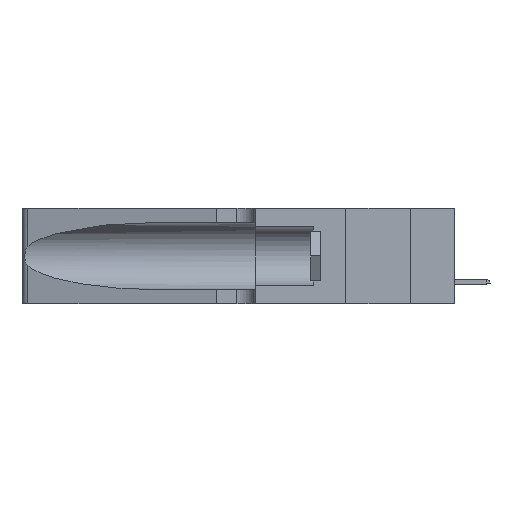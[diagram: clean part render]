
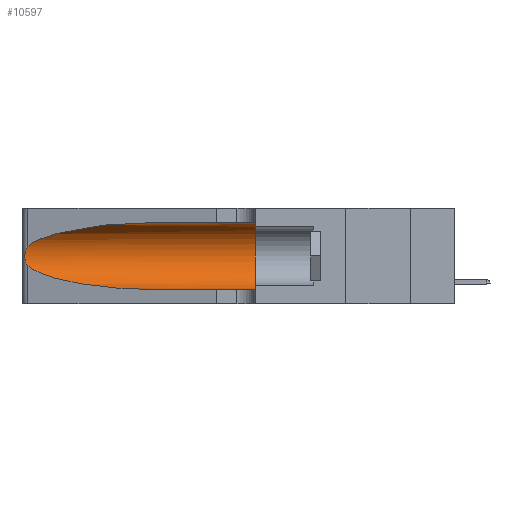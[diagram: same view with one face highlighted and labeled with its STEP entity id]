
A CAD part, left-side view. The second image highlights one B-rep face of the part: STEP entity #10597.
In plain terms, the highlighted cylindrical face has radius 3.308 mm (diameter 6.617 mm), a partial arc.
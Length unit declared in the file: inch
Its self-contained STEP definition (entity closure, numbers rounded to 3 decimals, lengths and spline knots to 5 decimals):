
#1844 = ORIENTED_EDGE ( 'NONE', *, *, #12029, .T. ) ;
#2015 = CARTESIAN_POINT ( 'NONE',  ( 0.25487, 1.22718, 0.22369 ) ) ;
#2252 = CARTESIAN_POINT ( 'NONE',  ( 0.26017, 1.23833, 0.17102 ) ) ;
#2272 = DIRECTION ( 'NONE',  ( 0., -1., 0. ) ) ;
#3058 =( BOUNDED_CURVE ( )  B_SPLINE_CURVE ( 3, ( #35166, #35877, #16623, #16371 ),
 .UNSPECIFIED., .F., .F. ) 
 B_SPLINE_CURVE_WITH_KNOTS ( ( 4, 4 ),
 ( 3.44316, 4.71239 ),
 .UNSPECIFIED. ) 
 CURVE ( )  GEOMETRIC_REPRESENTATION_ITEM ( )  RATIONAL_B_SPLINE_CURVE ( ( 1., 0.87, 0.87, 1. ) ) 
 REPRESENTATION_ITEM ( '' )  );
#3721 = DIRECTION ( 'NONE',  ( 0., 0., -1. ) ) ;
#3749 = EDGE_CURVE ( 'NONE', #28624, #7255, #40687, .T. ) ;
#4473 = CARTESIAN_POINT ( 'NONE',  ( 0.25487, 1.22718, 0.22369 ) ) ;
#4740 = CARTESIAN_POINT ( 'NONE',  ( 0.25487, 1.22718, 0.14631 ) ) ;
#5565 = AXIS2_PLACEMENT_3D ( 'NONE', #10467, #25495, #40591 ) ;
#5703 = EDGE_CURVE ( 'NONE', #43913, #32216, #21522, .T. ) ;
#6181 = AXIS2_PLACEMENT_3D ( 'NONE', #15055, #29634, #3721 ) ;
#6651 = CARTESIAN_POINT ( 'NONE',  ( 0.1305, 0.35, 0.05475 ) ) ;
#6897 = EDGE_CURVE ( 'NONE', #7255, #42079, #3058, .T. ) ;
#7200 = CIRCLE ( 'NONE', #5565, 0.13025 ) ;
#7255 = VERTEX_POINT ( 'NONE', #4740 ) ;
#9698 = CARTESIAN_POINT ( 'NONE',  ( 0.25854, 1.2359, 0.20912 ) ) ;
#9940 = CARTESIAN_POINT ( 'NONE',  ( 0.25555, 1.22993, 0.14849 ) ) ;
#10467 = CARTESIAN_POINT ( 'NONE',  ( 0.1305, 0.35, 0.185 ) ) ;
#10597 = ADVANCED_FACE ( 'NONE', ( #14576 ), #15294, .F. ) ;
#10708 = CARTESIAN_POINT ( 'NONE',  ( 0.1305, 1.61858, 0.31525 ) ) ;
#11825 = CARTESIAN_POINT ( 'NONE',  ( 0.2373, 1.15595, 0.28018 ) ) ;
#12029 = EDGE_CURVE ( 'NONE', #42079, #45597, #19730, .T. ) ;
#12962 = VECTOR ( 'NONE', #2272, 39.37008 ) ;
#14576 = FACE_OUTER_BOUND ( 'NONE', #19573, .T. ) ;
#15055 = CARTESIAN_POINT ( 'NONE',  ( 0.1305, 1.61858, 0.185 ) ) ;
#15294 = CYLINDRICAL_SURFACE ( 'NONE', #6181, 0.13025 ) ;
#16371 = CARTESIAN_POINT ( 'NONE',  ( 0.1305, 0.72297, 0.05475 ) ) ;
#16623 = CARTESIAN_POINT ( 'NONE',  ( 0.18966, 0.96281, 0.05475 ) ) ;
#17072 = CARTESIAN_POINT ( 'NONE',  ( 0.25555, 1.22994, 0.2215 ) ) ;
#17310 = CARTESIAN_POINT ( 'NONE',  ( 0.25856, 1.23593, 0.16098 ) ) ;
#18193 =( BOUNDED_CURVE ( )  B_SPLINE_CURVE ( 3, ( #45655, #19480, #11825, #42681 ),
 .UNSPECIFIED., .F., .F. ) 
 B_SPLINE_CURVE_WITH_KNOTS ( ( 4, 4 ),
 ( 1.5708, 2.84003 ),
 .UNSPECIFIED. ) 
 CURVE ( )  GEOMETRIC_REPRESENTATION_ITEM ( )  RATIONAL_B_SPLINE_CURVE ( ( 1., 0.87, 0.87, 1. ) ) 
 REPRESENTATION_ITEM ( '' )  );
#19480 = CARTESIAN_POINT ( 'NONE',  ( 0.18966, 0.96281, 0.31525 ) ) ;
#19573 = EDGE_LOOP ( 'NONE', ( #44862, #40835, #47446, #1844, #34543, #25046 ) ) ;
#19730 = LINE ( 'NONE', #23895, #36203 ) ;
#21243 = CARTESIAN_POINT ( 'NONE',  ( 0.26075, 1.23896, 0.178 ) ) ;
#21522 = LINE ( 'NONE', #10708, #12962 ) ;
#23460 = CARTESIAN_POINT ( 'NONE',  ( 0.1305, 0.35, 0.31525 ) ) ;
#23895 = CARTESIAN_POINT ( 'NONE',  ( 0.1305, 1.61858, 0.05475 ) ) ;
#24706 = CARTESIAN_POINT ( 'NONE',  ( 0.26018, 1.23835, 0.19895 ) ) ;
#24961 = CARTESIAN_POINT ( 'NONE',  ( 0.25487, 1.22718, 0.14631 ) ) ;
#25046 = ORIENTED_EDGE ( 'NONE', *, *, #5703, .F. ) ;
#25495 = DIRECTION ( 'NONE',  ( 0., 1., 0. ) ) ;
#28624 = VERTEX_POINT ( 'NONE', #4473 ) ;
#28661 = CARTESIAN_POINT ( 'NONE',  ( 0.25789, 1.23486, 0.15765 ) ) ;
#29634 = DIRECTION ( 'NONE',  ( 0., -1., 0. ) ) ;
#31303 = DIRECTION ( 'NONE',  ( 0., -1., 0. ) ) ;
#32092 = CARTESIAN_POINT ( 'NONE',  ( 0.25787, 1.23484, 0.2124 ) ) ;
#32109 = EDGE_CURVE ( 'NONE', #32216, #45597, #7200, .T. ) ;
#32216 = VERTEX_POINT ( 'NONE', #23460 ) ;
#33693 = EDGE_CURVE ( 'NONE', #43913, #28624, #18193, .T. ) ;
#34543 = ORIENTED_EDGE ( 'NONE', *, *, #32109, .F. ) ;
#35166 = CARTESIAN_POINT ( 'NONE',  ( 0.25487, 1.22718, 0.14631 ) ) ;
#35877 = CARTESIAN_POINT ( 'NONE',  ( 0.2373, 1.15595, 0.08982 ) ) ;
#36203 = VECTOR ( 'NONE', #31303, 39.37008 ) ;
#38674 = CARTESIAN_POINT ( 'NONE',  ( 0.1305, 0.72297, 0.31525 ) ) ;
#39793 = CARTESIAN_POINT ( 'NONE',  ( 0.26075, 1.23896, 0.19203 ) ) ;
#40591 = DIRECTION ( 'NONE',  ( 0., 0., 1. ) ) ;
#40687 = B_SPLINE_CURVE_WITH_KNOTS ( 'NONE', 3,
 ( #2015, #17072, #43503, #32092, #9698, #24706, #39793, #21243, #2252, #17310, #28661, #43751, #9940, #24961 ),
 .UNSPECIFIED., .F., .F.,
 ( 4, 2, 2, 2, 2, 2, 4 ),
 ( 0., 0.00027, 0.00053, 0.00107, 0.0016, 0.00187, 0.00214 ),
 .UNSPECIFIED. ) ;
#40835 = ORIENTED_EDGE ( 'NONE', *, *, #3749, .T. ) ;
#42079 = VERTEX_POINT ( 'NONE', #42188 ) ;
#42188 = CARTESIAN_POINT ( 'NONE',  ( 0.1305, 0.72297, 0.05475 ) ) ;
#42681 = CARTESIAN_POINT ( 'NONE',  ( 0.25487, 1.22718, 0.22369 ) ) ;
#43503 = CARTESIAN_POINT ( 'NONE',  ( 0.25639, 1.23184, 0.21858 ) ) ;
#43751 = CARTESIAN_POINT ( 'NONE',  ( 0.25639, 1.23186, 0.15144 ) ) ;
#43913 = VERTEX_POINT ( 'NONE', #38674 ) ;
#44862 = ORIENTED_EDGE ( 'NONE', *, *, #33693, .T. ) ;
#45597 = VERTEX_POINT ( 'NONE', #6651 ) ;
#45655 = CARTESIAN_POINT ( 'NONE',  ( 0.1305, 0.72297, 0.31525 ) ) ;
#47446 = ORIENTED_EDGE ( 'NONE', *, *, #6897, .T. ) ;
